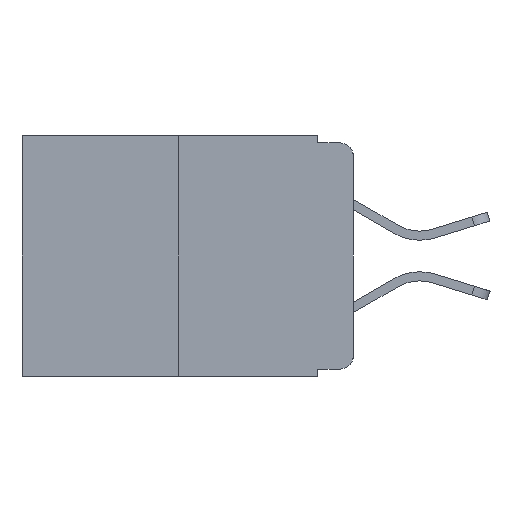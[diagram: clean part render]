
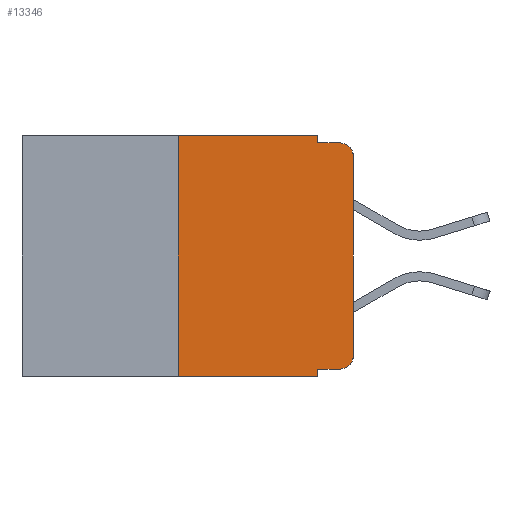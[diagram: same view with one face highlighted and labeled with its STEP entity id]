
A CAD part, left-side view. The second image highlights one B-rep face of the part: STEP entity #13346.
In plain terms, the highlighted planar face has unit normal (-1, 0, 0).
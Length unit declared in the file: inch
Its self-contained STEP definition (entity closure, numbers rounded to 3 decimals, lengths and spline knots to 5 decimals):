
#15 = LINE ( 'NONE', #4323, #12468 ) ;
#83 = CARTESIAN_POINT ( 'NONE',  ( 0., 0.051, -0.01 ) ) ;
#109 = EDGE_CURVE ( 'NONE', #5430, #13028, #6173, .T. ) ;
#138 = EDGE_CURVE ( 'NONE', #9168, #8818, #9963, .T. ) ;
#233 = ORIENTED_EDGE ( 'NONE', *, *, #8801, .F. ) ;
#477 = LINE ( 'NONE', #9012, #5546 ) ;
#636 = CARTESIAN_POINT ( 'NONE',  ( 0., 0., -0.03 ) ) ;
#904 = ORIENTED_EDGE ( 'NONE', *, *, #13666, .F. ) ;
#1084 = VERTEX_POINT ( 'NONE', #3897 ) ;
#1102 = VECTOR ( 'NONE', #8111, 39.37008 ) ;
#1139 = CARTESIAN_POINT ( 'NONE',  ( 0., 0.02, -0.313 ) ) ;
#1443 = EDGE_CURVE ( 'NONE', #4978, #3472, #3963, .T. ) ;
#1487 = EDGE_LOOP ( 'NONE', ( #9437, #13848, #904, #6664, #7830, #233, #7609, #11529, #8745, #4179 ) ) ;
#1977 = FACE_OUTER_BOUND ( 'NONE', #1487, .T. ) ;
#2040 = DIRECTION ( 'NONE',  ( 0., 0., -1. ) ) ;
#2122 = EDGE_CURVE ( 'NONE', #1084, #3472, #5142, .T. ) ;
#2456 = EDGE_CURVE ( 'NONE', #8001, #5430, #15, .T. ) ;
#2540 = LINE ( 'NONE', #13710, #9874 ) ;
#3111 = DIRECTION ( 'NONE',  ( 0., 0., 1. ) ) ;
#3197 = DIRECTION ( 'NONE',  ( 0., 0., 1. ) ) ;
#3461 = DIRECTION ( 'NONE',  ( 0., 0., -1. ) ) ;
#3472 = VERTEX_POINT ( 'NONE', #8419 ) ;
#3587 = CIRCLE ( 'NONE', #4426, 0.02 ) ;
#3801 = VECTOR ( 'NONE', #13355, 39.37008 ) ;
#3854 = DIRECTION ( 'NONE',  ( 0., -1., 0. ) ) ;
#3897 = CARTESIAN_POINT ( 'NONE',  ( 0., 0.25, -0.343 ) ) ;
#3963 = LINE ( 'NONE', #11377, #1102 ) ;
#4179 = ORIENTED_EDGE ( 'NONE', *, *, #8893, .T. ) ;
#4284 = CARTESIAN_POINT ( 'NONE',  ( 0., 0.051, 0. ) ) ;
#4323 = CARTESIAN_POINT ( 'NONE',  ( 0., 0., 0. ) ) ;
#4426 = AXIS2_PLACEMENT_3D ( 'NONE', #1139, #8869, #8739 ) ;
#4946 = CARTESIAN_POINT ( 'NONE',  ( 0., 0.051, -0.01 ) ) ;
#4978 = VERTEX_POINT ( 'NONE', #6081 ) ;
#5029 = EDGE_CURVE ( 'NONE', #4978, #10877, #2540, .T. ) ;
#5142 = LINE ( 'NONE', #8097, #8560 ) ;
#5276 = EDGE_CURVE ( 'NONE', #8818, #14081, #477, .T. ) ;
#5430 = VERTEX_POINT ( 'NONE', #636 ) ;
#5546 = VECTOR ( 'NONE', #13453, 39.37008 ) ;
#5643 = CARTESIAN_POINT ( 'NONE',  ( 0., 0.473, 0. ) ) ;
#6013 = DIRECTION ( 'NONE',  ( 0., -1., 0. ) ) ;
#6081 = CARTESIAN_POINT ( 'NONE',  ( 0., 0.051, -0.333 ) ) ;
#6173 = CIRCLE ( 'NONE', #11474, 0.02 ) ;
#6664 = ORIENTED_EDGE ( 'NONE', *, *, #5276, .F. ) ;
#7028 = CARTESIAN_POINT ( 'NONE',  ( 0., 0.25, 0. ) ) ;
#7152 = CARTESIAN_POINT ( 'NONE',  ( 0., 0.02, -0.01 ) ) ;
#7609 = ORIENTED_EDGE ( 'NONE', *, *, #2122, .T. ) ;
#7805 = CARTESIAN_POINT ( 'NONE',  ( 0., 0.02, -0.03 ) ) ;
#7830 = ORIENTED_EDGE ( 'NONE', *, *, #138, .F. ) ;
#8001 = VERTEX_POINT ( 'NONE', #13580 ) ;
#8097 = CARTESIAN_POINT ( 'NONE',  ( 0., 0.473, -0.343 ) ) ;
#8111 = DIRECTION ( 'NONE',  ( 0., 0., -1. ) ) ;
#8419 = CARTESIAN_POINT ( 'NONE',  ( 0., 0.051, -0.343 ) ) ;
#8560 = VECTOR ( 'NONE', #3854, 39.37008 ) ;
#8646 = PLANE ( 'NONE',  #9615 ) ;
#8739 = DIRECTION ( 'NONE',  ( 0., 0., -1. ) ) ;
#8745 = ORIENTED_EDGE ( 'NONE', *, *, #5029, .T. ) ;
#8801 = EDGE_CURVE ( 'NONE', #1084, #9168, #9068, .T. ) ;
#8818 = VERTEX_POINT ( 'NONE', #4284 ) ;
#8869 = DIRECTION ( 'NONE',  ( -1., 0., 0. ) ) ;
#8893 = EDGE_CURVE ( 'NONE', #10877, #8001, #3587, .T. ) ;
#9012 = CARTESIAN_POINT ( 'NONE',  ( 0., 0.051, 0. ) ) ;
#9068 = LINE ( 'NONE', #11757, #9769 ) ;
#9168 = VERTEX_POINT ( 'NONE', #7028 ) ;
#9376 = DIRECTION ( 'NONE',  ( 0., -1., 0. ) ) ;
#9437 = ORIENTED_EDGE ( 'NONE', *, *, #2456, .T. ) ;
#9615 = AXIS2_PLACEMENT_3D ( 'NONE', #11895, #11808, #2040 ) ;
#9769 = VECTOR ( 'NONE', #3111, 39.37008 ) ;
#9874 = VECTOR ( 'NONE', #9376, 39.37008 ) ;
#9963 = LINE ( 'NONE', #5643, #3801 ) ;
#10877 = VERTEX_POINT ( 'NONE', #11451 ) ;
#11377 = CARTESIAN_POINT ( 'NONE',  ( 0., 0.051, 0. ) ) ;
#11451 = CARTESIAN_POINT ( 'NONE',  ( 0., 0.02, -0.333 ) ) ;
#11474 = AXIS2_PLACEMENT_3D ( 'NONE', #7805, #13310, #3461 ) ;
#11529 = ORIENTED_EDGE ( 'NONE', *, *, #1443, .F. ) ;
#11757 = CARTESIAN_POINT ( 'NONE',  ( 0., 0.25, 0. ) ) ;
#11808 = DIRECTION ( 'NONE',  ( 1., 0., 0. ) ) ;
#11895 = CARTESIAN_POINT ( 'NONE',  ( 0., 0.473, 0. ) ) ;
#12468 = VECTOR ( 'NONE', #3197, 39.37008 ) ;
#12695 = VECTOR ( 'NONE', #6013, 39.37008 ) ;
#13028 = VERTEX_POINT ( 'NONE', #7152 ) ;
#13045 = LINE ( 'NONE', #4946, #12695 ) ;
#13310 = DIRECTION ( 'NONE',  ( -1., 0., 0. ) ) ;
#13346 = ADVANCED_FACE ( 'NONE', ( #1977 ), #8646, .F. ) ;
#13355 = DIRECTION ( 'NONE',  ( 0., -1., 0. ) ) ;
#13453 = DIRECTION ( 'NONE',  ( 0., 0., -1. ) ) ;
#13580 = CARTESIAN_POINT ( 'NONE',  ( 0., 0., -0.313 ) ) ;
#13666 = EDGE_CURVE ( 'NONE', #14081, #13028, #13045, .T. ) ;
#13710 = CARTESIAN_POINT ( 'NONE',  ( 0., 0.051, -0.333 ) ) ;
#13848 = ORIENTED_EDGE ( 'NONE', *, *, #109, .T. ) ;
#14081 = VERTEX_POINT ( 'NONE', #83 ) ;
